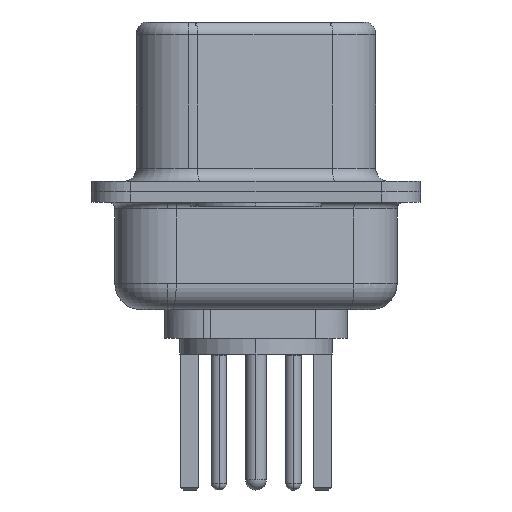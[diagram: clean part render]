
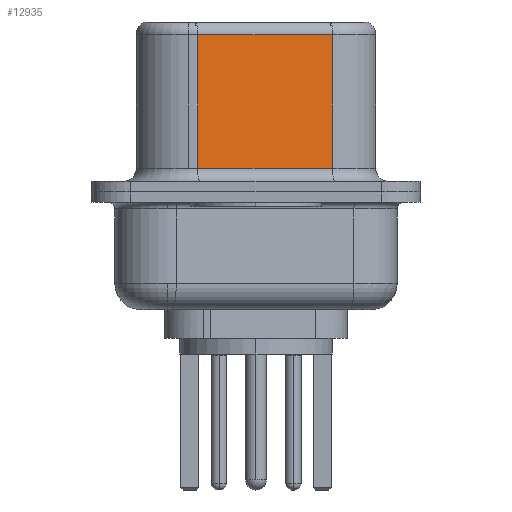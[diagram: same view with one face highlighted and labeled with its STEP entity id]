
A CAD part, left-side view. The second image highlights one B-rep face of the part: STEP entity #12935.
In plain terms, the highlighted planar face has unit normal (-0.985, -0.174, 0).
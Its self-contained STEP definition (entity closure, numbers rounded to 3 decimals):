
#287 = EDGE_CURVE ( 'NONE', #16855, #6982, #5188, .T. ) ;
#649 = CARTESIAN_POINT ( 'NONE',  ( 4.58, -2.927, 6.52 ) ) ;
#685 = CARTESIAN_POINT ( 'NONE',  ( 3.67, 2.233, 0.9 ) ) ;
#1994 = EDGE_CURVE ( 'NONE', #20668, #6022, #19080, .T. ) ;
#2519 = DIRECTION ( 'NONE',  ( -0.174, 0.985, 0. ) ) ;
#2761 = FACE_OUTER_BOUND ( 'NONE', #17760, .T. ) ;
#4194 = DIRECTION ( 'NONE',  ( -0.174, 0.985, 0. ) ) ;
#4499 = CARTESIAN_POINT ( 'NONE',  ( 4.58, -2.927, 0.9 ) ) ;
#5188 = LINE ( 'NONE', #4499, #10195 ) ;
#5310 = EDGE_CURVE ( 'NONE', #20668, #6982, #16941, .T. ) ;
#5333 = CARTESIAN_POINT ( 'NONE',  ( 4.58, -2.927, 6.02 ) ) ;
#5356 = VECTOR ( 'NONE', #12219, 1000. ) ;
#5633 = CARTESIAN_POINT ( 'NONE',  ( 3.67, 2.233, 6.02 ) ) ;
#6022 = VERTEX_POINT ( 'NONE', #5633 ) ;
#6355 = ORIENTED_EDGE ( 'NONE', *, *, #23865, .T. ) ;
#6982 = VERTEX_POINT ( 'NONE', #7998 ) ;
#7998 = CARTESIAN_POINT ( 'NONE',  ( 4.58, -2.927, 0.9 ) ) ;
#8217 = ORIENTED_EDGE ( 'NONE', *, *, #287, .T. ) ;
#9303 = ORIENTED_EDGE ( 'NONE', *, *, #5310, .F. ) ;
#9835 = ORIENTED_EDGE ( 'NONE', *, *, #1994, .T. ) ;
#10024 = PLANE ( 'NONE',  #14705 ) ;
#10195 = VECTOR ( 'NONE', #22407, 1000. ) ;
#10351 = LINE ( 'NONE', #19453, #5356 ) ;
#12219 = DIRECTION ( 'NONE',  ( 0., 0., -1. ) ) ;
#12935 = ADVANCED_FACE ( 'NONE', ( #2761 ), #10024, .F. ) ;
#13696 = VECTOR ( 'NONE', #4194, 1000. ) ;
#13765 = DIRECTION ( 'NONE',  ( 0.985, 0.174, 0. ) ) ;
#14655 = CARTESIAN_POINT ( 'NONE',  ( 4.58, -2.927, 6.52 ) ) ;
#14705 = AXIS2_PLACEMENT_3D ( 'NONE', #649, #13765, #2519 ) ;
#16855 = VERTEX_POINT ( 'NONE', #685 ) ;
#16941 = LINE ( 'NONE', #14655, #21197 ) ;
#17499 = CARTESIAN_POINT ( 'NONE',  ( 4.58, -2.927, 6.02 ) ) ;
#17760 = EDGE_LOOP ( 'NONE', ( #9303, #9835, #6355, #8217 ) ) ;
#19080 = LINE ( 'NONE', #17499, #13696 ) ;
#19453 = CARTESIAN_POINT ( 'NONE',  ( 3.67, 2.233, 6.52 ) ) ;
#19708 = DIRECTION ( 'NONE',  ( 0., 0., -1. ) ) ;
#20668 = VERTEX_POINT ( 'NONE', #5333 ) ;
#21197 = VECTOR ( 'NONE', #19708, 1000. ) ;
#22407 = DIRECTION ( 'NONE',  ( 0.174, -0.985, 0. ) ) ;
#23865 = EDGE_CURVE ( 'NONE', #6022, #16855, #10351, .T. ) ;
